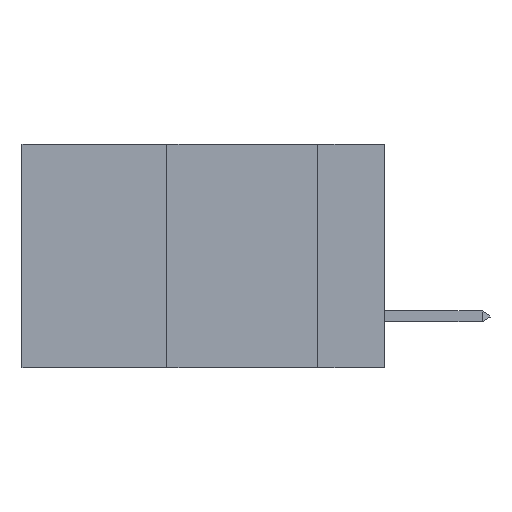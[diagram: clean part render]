
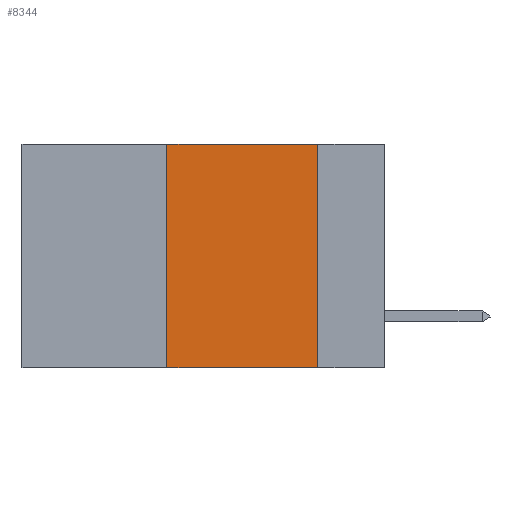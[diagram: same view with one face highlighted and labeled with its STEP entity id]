
A CAD part, left-side view. The second image highlights one B-rep face of the part: STEP entity #8344.
In plain terms, the highlighted planar face has unit normal (-1, 0, 0).
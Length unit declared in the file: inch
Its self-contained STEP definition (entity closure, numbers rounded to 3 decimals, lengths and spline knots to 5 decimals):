
#252 = AXIS2_PLACEMENT_3D ( 'NONE', #7780, #7835, #1208 ) ;
#292 = VERTEX_POINT ( 'NONE', #6001 ) ;
#462 = DIRECTION ( 'NONE',  ( 0., -1., 0. ) ) ;
#499 = VERTEX_POINT ( 'NONE', #3360 ) ;
#1125 = CARTESIAN_POINT ( 'NONE',  ( 0., 0.6, 0. ) ) ;
#1208 = DIRECTION ( 'NONE',  ( 0., 0., -1. ) ) ;
#1330 = CARTESIAN_POINT ( 'NONE',  ( 0., 0.11, 0. ) ) ;
#1543 = VERTEX_POINT ( 'NONE', #10557 ) ;
#1707 = ORIENTED_EDGE ( 'NONE', *, *, #10312, .T. ) ;
#1728 = VECTOR ( 'NONE', #462, 39.37008 ) ;
#1995 = VECTOR ( 'NONE', #5161, 39.37008 ) ;
#2031 = PLANE ( 'NONE',  #252 ) ;
#2239 = DIRECTION ( 'NONE',  ( 0., 0., -1. ) ) ;
#2439 = ORIENTED_EDGE ( 'NONE', *, *, #3418, .F. ) ;
#2567 = CARTESIAN_POINT ( 'NONE',  ( 0., 0.36, 0. ) ) ;
#3118 = VERTEX_POINT ( 'NONE', #1330 ) ;
#3360 = CARTESIAN_POINT ( 'NONE',  ( 0., 0.11, -0.37 ) ) ;
#3418 = EDGE_CURVE ( 'NONE', #292, #3118, #3920, .T. ) ;
#3920 = LINE ( 'NONE', #1125, #1728 ) ;
#4672 = EDGE_LOOP ( 'NONE', ( #9172, #2439, #6078, #1707 ) ) ;
#5070 = EDGE_CURVE ( 'NONE', #1543, #292, #7532, .T. ) ;
#5161 = DIRECTION ( 'NONE',  ( 0., 0., 1. ) ) ;
#5208 = FACE_OUTER_BOUND ( 'NONE', #4672, .T. ) ;
#5226 = CARTESIAN_POINT ( 'NONE',  ( 0., 0.6, -0.37 ) ) ;
#5569 = CARTESIAN_POINT ( 'NONE',  ( 0., 0.11, 0. ) ) ;
#6001 = CARTESIAN_POINT ( 'NONE',  ( 0., 0.36, 0. ) ) ;
#6078 = ORIENTED_EDGE ( 'NONE', *, *, #5070, .F. ) ;
#6150 = VECTOR ( 'NONE', #10341, 39.37008 ) ;
#7532 = LINE ( 'NONE', #2567, #1995 ) ;
#7780 = CARTESIAN_POINT ( 'NONE',  ( 0., 0.6, 0. ) ) ;
#7835 = DIRECTION ( 'NONE',  ( 1., 0., 0. ) ) ;
#8285 = LINE ( 'NONE', #5226, #6150 ) ;
#8344 = ADVANCED_FACE ( 'NONE', ( #5208 ), #2031, .F. ) ;
#8947 = VECTOR ( 'NONE', #2239, 39.37008 ) ;
#9172 = ORIENTED_EDGE ( 'NONE', *, *, #9837, .F. ) ;
#9837 = EDGE_CURVE ( 'NONE', #3118, #499, #10253, .T. ) ;
#10253 = LINE ( 'NONE', #5569, #8947 ) ;
#10312 = EDGE_CURVE ( 'NONE', #1543, #499, #8285, .T. ) ;
#10341 = DIRECTION ( 'NONE',  ( 0., -1., 0. ) ) ;
#10557 = CARTESIAN_POINT ( 'NONE',  ( 0., 0.36, -0.37 ) ) ;
